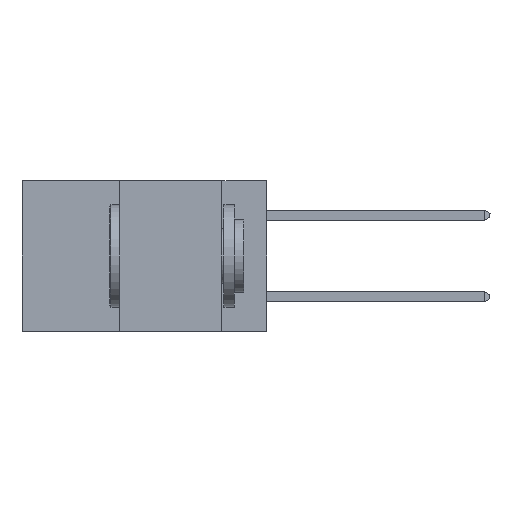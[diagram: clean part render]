
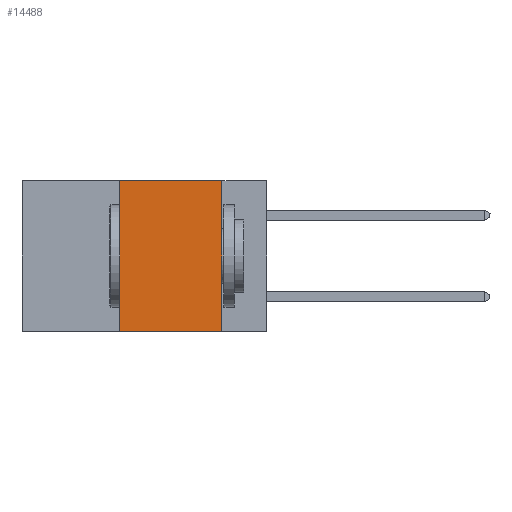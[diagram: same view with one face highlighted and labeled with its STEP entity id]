
A CAD part, left-side view. The second image highlights one B-rep face of the part: STEP entity #14488.
In plain terms, the highlighted planar face has unit normal (-1, 0, 0).
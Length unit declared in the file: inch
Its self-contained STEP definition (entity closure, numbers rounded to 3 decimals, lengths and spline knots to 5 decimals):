
#242 = CARTESIAN_POINT ( 'NONE',  ( 0., 0.6, 0. ) ) ;
#315 = DIRECTION ( 'NONE',  ( 0., 0., -1. ) ) ;
#677 = VERTEX_POINT ( 'NONE', #1695 ) ;
#1594 = CARTESIAN_POINT ( 'NONE',  ( 0., 0.36, 0. ) ) ;
#1695 = CARTESIAN_POINT ( 'NONE',  ( 0., 0.11, 0. ) ) ;
#2062 = LINE ( 'NONE', #6075, #13741 ) ;
#2217 = CARTESIAN_POINT ( 'NONE',  ( 0., 0.6, -0.37 ) ) ;
#2991 = VERTEX_POINT ( 'NONE', #14189 ) ;
#3220 = CARTESIAN_POINT ( 'NONE',  ( 0., 0.36, 0. ) ) ;
#3274 = DIRECTION ( 'NONE',  ( 0., 0., 1. ) ) ;
#4047 = FACE_OUTER_BOUND ( 'NONE', #12940, .T. ) ;
#4329 = CARTESIAN_POINT ( 'NONE',  ( 0., 0.11, 0. ) ) ;
#4603 = EDGE_CURVE ( 'NONE', #5359, #2991, #10371, .T. ) ;
#5359 = VERTEX_POINT ( 'NONE', #10878 ) ;
#5666 = LINE ( 'NONE', #3220, #14746 ) ;
#6075 = CARTESIAN_POINT ( 'NONE',  ( 0., 0.6, 0. ) ) ;
#6242 = DIRECTION ( 'NONE',  ( 1., 0., 0. ) ) ;
#9296 = DIRECTION ( 'NONE',  ( 0., 0., -1. ) ) ;
#9323 = EDGE_CURVE ( 'NONE', #677, #2991, #14584, .T. ) ;
#9679 = ORIENTED_EDGE ( 'NONE', *, *, #12509, .F. ) ;
#9858 = PLANE ( 'NONE',  #13064 ) ;
#10371 = LINE ( 'NONE', #2217, #12299 ) ;
#10627 = EDGE_CURVE ( 'NONE', #5359, #11754, #5666, .T. ) ;
#10878 = CARTESIAN_POINT ( 'NONE',  ( 0., 0.36, -0.37 ) ) ;
#11358 = VECTOR ( 'NONE', #9296, 39.37008 ) ;
#11754 = VERTEX_POINT ( 'NONE', #1594 ) ;
#12299 = VECTOR ( 'NONE', #14227, 39.37008 ) ;
#12509 = EDGE_CURVE ( 'NONE', #11754, #677, #2062, .T. ) ;
#12940 = EDGE_LOOP ( 'NONE', ( #15302, #9679, #14258, #14906 ) ) ;
#13064 = AXIS2_PLACEMENT_3D ( 'NONE', #242, #6242, #315 ) ;
#13741 = VECTOR ( 'NONE', #14417, 39.37008 ) ;
#14189 = CARTESIAN_POINT ( 'NONE',  ( 0., 0.11, -0.37 ) ) ;
#14227 = DIRECTION ( 'NONE',  ( 0., -1., 0. ) ) ;
#14258 = ORIENTED_EDGE ( 'NONE', *, *, #10627, .F. ) ;
#14417 = DIRECTION ( 'NONE',  ( 0., -1., 0. ) ) ;
#14488 = ADVANCED_FACE ( 'NONE', ( #4047 ), #9858, .F. ) ;
#14584 = LINE ( 'NONE', #4329, #11358 ) ;
#14746 = VECTOR ( 'NONE', #3274, 39.37008 ) ;
#14906 = ORIENTED_EDGE ( 'NONE', *, *, #4603, .T. ) ;
#15302 = ORIENTED_EDGE ( 'NONE', *, *, #9323, .F. ) ;
